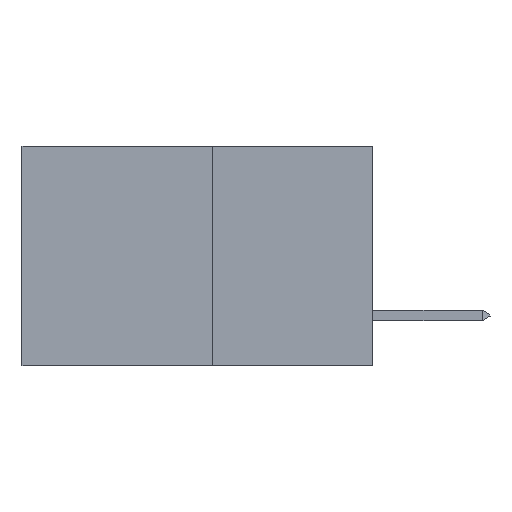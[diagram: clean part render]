
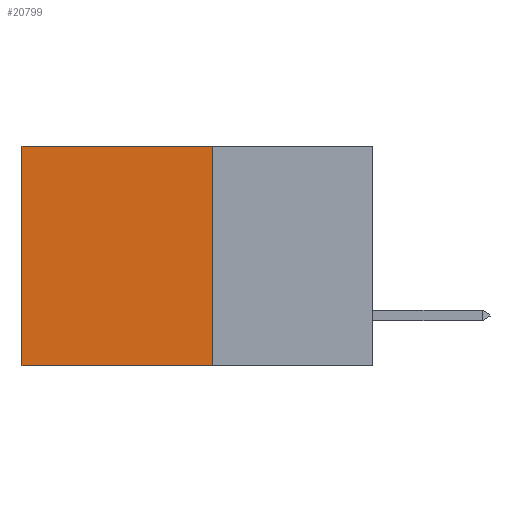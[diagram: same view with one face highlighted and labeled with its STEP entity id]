
A CAD part, left-side view. The second image highlights one B-rep face of the part: STEP entity #20799.
In plain terms, the highlighted planar face has unit normal (-1, 0, 0).
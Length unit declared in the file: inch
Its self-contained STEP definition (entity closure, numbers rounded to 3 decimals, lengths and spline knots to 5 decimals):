
#520 = ORIENTED_EDGE ( 'NONE', *, *, #8861, .F. ) ;
#3081 = VERTEX_POINT ( 'NONE', #3706 ) ;
#3592 = ORIENTED_EDGE ( 'NONE', *, *, #9422, .T. ) ;
#3706 = CARTESIAN_POINT ( 'NONE',  ( 0.277, 0.59, -0.37 ) ) ;
#4119 = CARTESIAN_POINT ( 'NONE',  ( 0.277, 0.27, 0. ) ) ;
#4977 = CARTESIAN_POINT ( 'NONE',  ( 0.277, 0.27, -0.37 ) ) ;
#5083 = EDGE_CURVE ( 'NONE', #20285, #6802, #18174, .T. ) ;
#6802 = VERTEX_POINT ( 'NONE', #7118 ) ;
#7118 = CARTESIAN_POINT ( 'NONE',  ( 0.277, 0.27, -0.37 ) ) ;
#8341 = DIRECTION ( 'NONE',  ( 0., 0., -1. ) ) ;
#8861 = EDGE_CURVE ( 'NONE', #6802, #3081, #13958, .T. ) ;
#9320 = PLANE ( 'NONE',  #9527 ) ;
#9422 = EDGE_CURVE ( 'NONE', #14948, #3081, #19440, .T. ) ;
#9527 = AXIS2_PLACEMENT_3D ( 'NONE', #21064, #11295, #24964 ) ;
#9886 = FACE_OUTER_BOUND ( 'NONE', #12411, .T. ) ;
#11079 = LINE ( 'NONE', #4119, #25447 ) ;
#11287 = EDGE_CURVE ( 'NONE', #20285, #14948, #11079, .T. ) ;
#11295 = DIRECTION ( 'NONE',  ( 1., 0., 0. ) ) ;
#12411 = EDGE_LOOP ( 'NONE', ( #3592, #520, #25484, #19501 ) ) ;
#12956 = VECTOR ( 'NONE', #8341, 39.37008 ) ;
#13006 = CARTESIAN_POINT ( 'NONE',  ( 0.277, 0.59, -0.37 ) ) ;
#13958 = LINE ( 'NONE', #4977, #22535 ) ;
#14948 = VERTEX_POINT ( 'NONE', #19507 ) ;
#15415 = CARTESIAN_POINT ( 'NONE',  ( 0.277, 0.27, 0. ) ) ;
#18174 = LINE ( 'NONE', #18777, #12956 ) ;
#18777 = CARTESIAN_POINT ( 'NONE',  ( 0.277, 0.27, -0.37 ) ) ;
#18826 = DIRECTION ( 'NONE',  ( 0., 0., -1. ) ) ;
#19440 = LINE ( 'NONE', #13006, #20063 ) ;
#19501 = ORIENTED_EDGE ( 'NONE', *, *, #11287, .T. ) ;
#19507 = CARTESIAN_POINT ( 'NONE',  ( 0.277, 0.59, 0. ) ) ;
#20063 = VECTOR ( 'NONE', #18826, 39.37008 ) ;
#20285 = VERTEX_POINT ( 'NONE', #15415 ) ;
#20799 = ADVANCED_FACE ( 'NONE', ( #9886 ), #9320, .F. ) ;
#21064 = CARTESIAN_POINT ( 'NONE',  ( 0.277, 0.27, -0.37 ) ) ;
#21915 = DIRECTION ( 'NONE',  ( 0., 1., 0. ) ) ;
#22535 = VECTOR ( 'NONE', #24660, 39.37008 ) ;
#24660 = DIRECTION ( 'NONE',  ( 0., 1., 0. ) ) ;
#24964 = DIRECTION ( 'NONE',  ( 0., 0., -1. ) ) ;
#25447 = VECTOR ( 'NONE', #21915, 39.37008 ) ;
#25484 = ORIENTED_EDGE ( 'NONE', *, *, #5083, .F. ) ;
